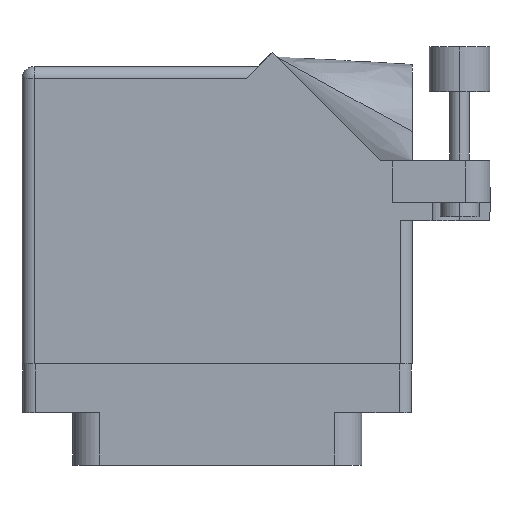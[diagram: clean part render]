
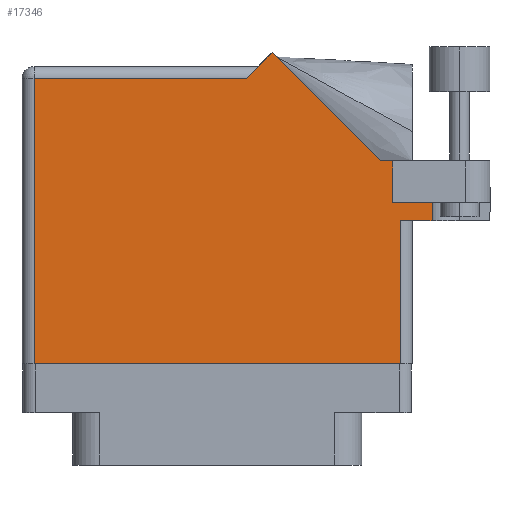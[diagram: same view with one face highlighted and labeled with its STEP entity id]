
A CAD part, front view. The second image highlights one B-rep face of the part: STEP entity #17346.
In plain terms, the highlighted face is planar.
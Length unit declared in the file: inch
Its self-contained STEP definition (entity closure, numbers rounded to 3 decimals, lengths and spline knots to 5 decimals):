
#246 = CARTESIAN_POINT ( 'NONE',  ( 0.943, 0.637, 0.455 ) ) ;
#308 = ORIENTED_EDGE ( 'NONE', *, *, #22306, .T. ) ;
#324 = LINE ( 'NONE', #22848, #24884 ) ;
#422 = VECTOR ( 'NONE', #14067, 39.37008 ) ;
#622 = DIRECTION ( 'NONE',  ( 0., 0., -1. ) ) ;
#1024 = EDGE_CURVE ( 'NONE', #19025, #23368, #26605, .T. ) ;
#1050 = VECTOR ( 'NONE', #4188, 39.37008 ) ;
#1081 = CARTESIAN_POINT ( 'NONE',  ( -0.943, -0.1, 0.455 ) ) ;
#1233 = VERTEX_POINT ( 'NONE', #22448 ) ;
#1960 = DIRECTION ( 'NONE',  ( 0., -1., 0. ) ) ;
#2042 = VERTEX_POINT ( 'NONE', #1081 ) ;
#2281 = CARTESIAN_POINT ( 'NONE',  ( 0.905, 0.731, 0.455 ) ) ;
#2844 = AXIS2_PLACEMENT_3D ( 'NONE', #25791, #622, #14603 ) ;
#4062 = VERTEX_POINT ( 'NONE', #23312 ) ;
#4188 = DIRECTION ( 'NONE',  ( -1., 0., 0. ) ) ;
#4431 = EDGE_CURVE ( 'NONE', #4062, #1233, #7873, .T. ) ;
#4652 = ORIENTED_EDGE ( 'NONE', *, *, #23906, .F. ) ;
#4743 = LINE ( 'NONE', #27610, #35040 ) ;
#5709 = DIRECTION ( 'NONE',  ( -1., 0., 0. ) ) ;
#5854 = LINE ( 'NONE', #8822, #29127 ) ;
#6744 = VECTOR ( 'NONE', #6768, 39.37008 ) ;
#6768 = DIRECTION ( 'NONE',  ( 1., 0., 0. ) ) ;
#7553 = DIRECTION ( 'NONE',  ( 0., -1., 0. ) ) ;
#7873 = LINE ( 'NONE', #9301, #422 ) ;
#8143 = FACE_OUTER_BOUND ( 'NONE', #9992, .T. ) ;
#8388 = EDGE_CURVE ( 'NONE', #26968, #10505, #26034, .T. ) ;
#8578 = EDGE_CURVE ( 'NONE', #1233, #26001, #30495, .T. ) ;
#8822 = CARTESIAN_POINT ( 'NONE',  ( 0.83942, 0.944, 0.455 ) ) ;
#9023 = CARTESIAN_POINT ( 'NONE',  ( 0.83942, 0.944, 0.455 ) ) ;
#9301 = CARTESIAN_POINT ( 'NONE',  ( 0.212, 1.43, 0.455 ) ) ;
#9393 = CARTESIAN_POINT ( 'NONE',  ( 0.905, 0.944, 0.455 ) ) ;
#9992 = EDGE_LOOP ( 'NONE', ( #12567, #16875, #27930, #4652, #20813, #308, #28002, #11455, #11710, #20968, #13511 ) ) ;
#10063 = CARTESIAN_POINT ( 'NONE',  ( 1.1065, 0.731, 0.455 ) ) ;
#10505 = VERTEX_POINT ( 'NONE', #10063 ) ;
#11311 = VERTEX_POINT ( 'NONE', #9393 ) ;
#11405 = DIRECTION ( 'NONE',  ( 1., 0., 0. ) ) ;
#11455 = ORIENTED_EDGE ( 'NONE', *, *, #19028, .T. ) ;
#11710 = ORIENTED_EDGE ( 'NONE', *, *, #4431, .T. ) ;
#12065 = CARTESIAN_POINT ( 'NONE',  ( 0.905, 0.731, 0.455 ) ) ;
#12468 = LINE ( 'NONE', #24034, #17252 ) ;
#12567 = ORIENTED_EDGE ( 'NONE', *, *, #21732, .T. ) ;
#13511 = ORIENTED_EDGE ( 'NONE', *, *, #26969, .T. ) ;
#14067 = DIRECTION ( 'NONE',  ( -0.707, -0.707, 0. ) ) ;
#14603 = DIRECTION ( 'NONE',  ( -1., 0., 0. ) ) ;
#14630 = VECTOR ( 'NONE', #32791, 39.37008 ) ;
#14696 = VERTEX_POINT ( 'NONE', #19317 ) ;
#14919 = DIRECTION ( 'NONE',  ( -0.707, 0.707, 0. ) ) ;
#15092 = CARTESIAN_POINT ( 'NONE',  ( 0.943, 0.637, 0.455 ) ) ;
#16094 = VECTOR ( 'NONE', #7553, 39.37008 ) ;
#16812 = VERTEX_POINT ( 'NONE', #9023 ) ;
#16875 = ORIENTED_EDGE ( 'NONE', *, *, #1024, .T. ) ;
#17252 = VECTOR ( 'NONE', #1960, 39.37008 ) ;
#17346 = ADVANCED_FACE ( 'NONE', ( #8143 ), #17400, .F. ) ;
#17400 = PLANE ( 'NONE',  #2844 ) ;
#18249 = CARTESIAN_POINT ( 'NONE',  ( -1.005, 1.368, 0.455 ) ) ;
#18810 = DIRECTION ( 'NONE',  ( 0., 1., 0. ) ) ;
#19025 = VERTEX_POINT ( 'NONE', #26000 ) ;
#19028 = EDGE_CURVE ( 'NONE', #16812, #4062, #5854, .T. ) ;
#19317 = CARTESIAN_POINT ( 'NONE',  ( 1.1065, 0.637, 0.455 ) ) ;
#20813 = ORIENTED_EDGE ( 'NONE', *, *, #8388, .F. ) ;
#20968 = ORIENTED_EDGE ( 'NONE', *, *, #8578, .T. ) ;
#20973 = DIRECTION ( 'NONE',  ( 0., 1., 0. ) ) ;
#21493 = CARTESIAN_POINT ( 'NONE',  ( 1.1065, 1.06177, 0.455 ) ) ;
#21732 = EDGE_CURVE ( 'NONE', #2042, #19025, #4743, .T. ) ;
#22306 = EDGE_CURVE ( 'NONE', #26968, #11311, #36311, .T. ) ;
#22448 = CARTESIAN_POINT ( 'NONE',  ( 0.15, 1.368, 0.455 ) ) ;
#22848 = CARTESIAN_POINT ( 'NONE',  ( 1.405, 0.944, 0.455 ) ) ;
#23312 = CARTESIAN_POINT ( 'NONE',  ( 0.28271, 1.50071, 0.455 ) ) ;
#23368 = VERTEX_POINT ( 'NONE', #246 ) ;
#23603 = LINE ( 'NONE', #21493, #16094 ) ;
#23862 = LINE ( 'NONE', #26990, #14630 ) ;
#23906 = EDGE_CURVE ( 'NONE', #10505, #14696, #23603, .T. ) ;
#24034 = CARTESIAN_POINT ( 'NONE',  ( -0.943, -0.1, 0.455 ) ) ;
#24884 = VECTOR ( 'NONE', #5709, 39.37008 ) ;
#25791 = CARTESIAN_POINT ( 'NONE',  ( -1.005, 1.43, 0.455 ) ) ;
#26000 = CARTESIAN_POINT ( 'NONE',  ( 0.943, -0.1, 0.455 ) ) ;
#26001 = VERTEX_POINT ( 'NONE', #27678 ) ;
#26034 = LINE ( 'NONE', #12065, #6744 ) ;
#26605 = LINE ( 'NONE', #15092, #27063 ) ;
#26968 = VERTEX_POINT ( 'NONE', #35222 ) ;
#26969 = EDGE_CURVE ( 'NONE', #26001, #2042, #12468, .T. ) ;
#26990 = CARTESIAN_POINT ( 'NONE',  ( 1.005, 0.637, 0.455 ) ) ;
#27024 = EDGE_CURVE ( 'NONE', #23368, #14696, #23862, .T. ) ;
#27063 = VECTOR ( 'NONE', #20973, 39.37008 ) ;
#27610 = CARTESIAN_POINT ( 'NONE',  ( -1.005, -0.1, 0.455 ) ) ;
#27678 = CARTESIAN_POINT ( 'NONE',  ( -0.943, 1.368, 0.455 ) ) ;
#27930 = ORIENTED_EDGE ( 'NONE', *, *, #27024, .T. ) ;
#28002 = ORIENTED_EDGE ( 'NONE', *, *, #31421, .T. ) ;
#29127 = VECTOR ( 'NONE', #14919, 39.37008 ) ;
#30495 = LINE ( 'NONE', #18249, #1050 ) ;
#31421 = EDGE_CURVE ( 'NONE', #11311, #16812, #324, .T. ) ;
#32791 = DIRECTION ( 'NONE',  ( 1., 0., 0. ) ) ;
#34620 = VECTOR ( 'NONE', #18810, 39.37008 ) ;
#35040 = VECTOR ( 'NONE', #11405, 39.37008 ) ;
#35222 = CARTESIAN_POINT ( 'NONE',  ( 0.905, 0.731, 0.455 ) ) ;
#36311 = LINE ( 'NONE', #2281, #34620 ) ;
